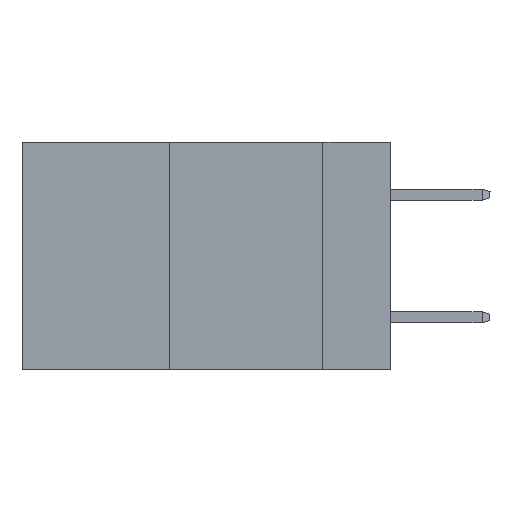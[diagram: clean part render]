
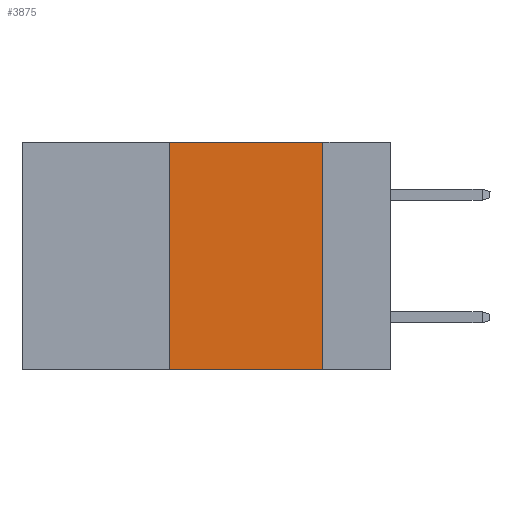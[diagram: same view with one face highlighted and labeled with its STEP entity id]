
A CAD part, left-side view. The second image highlights one B-rep face of the part: STEP entity #3875.
In plain terms, the highlighted planar face has unit normal (-1, 0, 0).
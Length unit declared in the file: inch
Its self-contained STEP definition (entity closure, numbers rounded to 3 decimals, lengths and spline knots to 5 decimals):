
#1504 = EDGE_CURVE ( 'NONE', #20724, #22955, #14804, .T. ) ;
#2368 = LINE ( 'NONE', #17550, #4955 ) ;
#2607 = ORIENTED_EDGE ( 'NONE', *, *, #16019, .F. ) ;
#2807 = DIRECTION ( 'NONE',  ( 0., -1., 0. ) ) ;
#3055 = ORIENTED_EDGE ( 'NONE', *, *, #10869, .F. ) ;
#3710 = VERTEX_POINT ( 'NONE', #23380 ) ;
#3812 = VECTOR ( 'NONE', #24830, 39.37008 ) ;
#3875 = ADVANCED_FACE ( 'NONE', ( #22092 ), #10810, .F. ) ;
#4955 = VECTOR ( 'NONE', #15766, 39.37008 ) ;
#5006 = EDGE_CURVE ( 'NONE', #3710, #22955, #2368, .T. ) ;
#5514 = CARTESIAN_POINT ( 'NONE',  ( 0., 0.11, -0.37 ) ) ;
#6456 = DIRECTION ( 'NONE',  ( 1., 0., 0. ) ) ;
#7266 = ORIENTED_EDGE ( 'NONE', *, *, #5006, .F. ) ;
#7739 = CARTESIAN_POINT ( 'NONE',  ( 0., 0.36, 0. ) ) ;
#7860 = CARTESIAN_POINT ( 'NONE',  ( 0., 0.36, -0.37 ) ) ;
#8214 = ORIENTED_EDGE ( 'NONE', *, *, #1504, .T. ) ;
#10621 = LINE ( 'NONE', #14801, #15527 ) ;
#10810 = PLANE ( 'NONE',  #20585 ) ;
#10869 = EDGE_CURVE ( 'NONE', #20724, #23045, #17151, .T. ) ;
#13141 = CARTESIAN_POINT ( 'NONE',  ( 0., 0.6, -0.37 ) ) ;
#14229 = DIRECTION ( 'NONE',  ( 0., 0., -1. ) ) ;
#14801 = CARTESIAN_POINT ( 'NONE',  ( 0., 0.6, 0. ) ) ;
#14804 = LINE ( 'NONE', #13141, #3812 ) ;
#15527 = VECTOR ( 'NONE', #2807, 39.37008 ) ;
#15766 = DIRECTION ( 'NONE',  ( 0., 0., -1. ) ) ;
#16019 = EDGE_CURVE ( 'NONE', #23045, #3710, #10621, .T. ) ;
#16523 = CARTESIAN_POINT ( 'NONE',  ( 0., 0.6, 0. ) ) ;
#17151 = LINE ( 'NONE', #7739, #19110 ) ;
#17550 = CARTESIAN_POINT ( 'NONE',  ( 0., 0.11, 0. ) ) ;
#19110 = VECTOR ( 'NONE', #21073, 39.37008 ) ;
#20585 = AXIS2_PLACEMENT_3D ( 'NONE', #16523, #6456, #14229 ) ;
#20724 = VERTEX_POINT ( 'NONE', #7860 ) ;
#21073 = DIRECTION ( 'NONE',  ( 0., 0., 1. ) ) ;
#21274 = CARTESIAN_POINT ( 'NONE',  ( 0., 0.36, 0. ) ) ;
#21999 = EDGE_LOOP ( 'NONE', ( #7266, #2607, #3055, #8214 ) ) ;
#22092 = FACE_OUTER_BOUND ( 'NONE', #21999, .T. ) ;
#22955 = VERTEX_POINT ( 'NONE', #5514 ) ;
#23045 = VERTEX_POINT ( 'NONE', #21274 ) ;
#23380 = CARTESIAN_POINT ( 'NONE',  ( 0., 0.11, 0. ) ) ;
#24830 = DIRECTION ( 'NONE',  ( 0., -1., 0. ) ) ;
